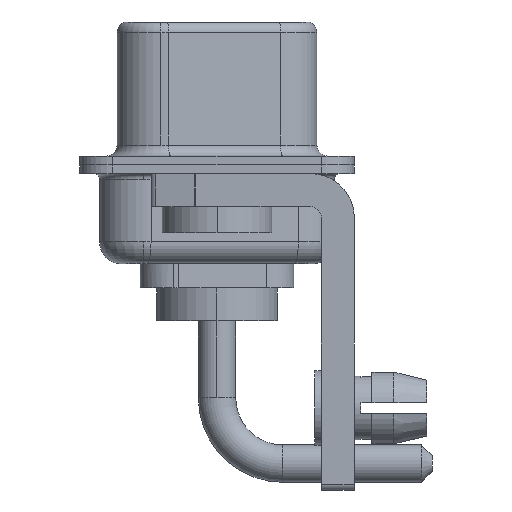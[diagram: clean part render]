
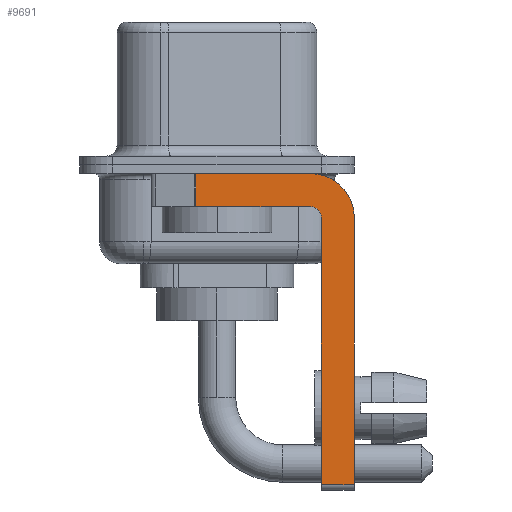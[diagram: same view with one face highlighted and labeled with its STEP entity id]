
A CAD part, left-side view. The second image highlights one B-rep face of the part: STEP entity #9691.
In plain terms, the highlighted planar face has unit normal (-1, 0, 0).
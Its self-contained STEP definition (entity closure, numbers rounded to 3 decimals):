
#87 = AXIS2_PLACEMENT_3D ( 'NONE', #12002, #17520, #7473 ) ;
#118 = AXIS2_PLACEMENT_3D ( 'NONE', #17825, #10925, #2314 ) ;
#551 = DIRECTION ( 'NONE',  ( 0., 0., 1. ) ) ;
#758 = CARTESIAN_POINT ( 'NONE',  ( -2.9, -4.25, -14.55 ) ) ;
#768 = AXIS2_PLACEMENT_3D ( 'NONE', #18091, #13930, #10912 ) ;
#1028 = CARTESIAN_POINT ( 'NONE',  ( -2.9, -6.25, -2.4 ) ) ;
#1079 = EDGE_CURVE ( 'NONE', #1593, #11810, #5171, .T. ) ;
#1318 = ORIENTED_EDGE ( 'NONE', *, *, #18041, .F. ) ;
#1593 = VERTEX_POINT ( 'NONE', #12363 ) ;
#2280 = CARTESIAN_POINT ( 'NONE',  ( -2.9, -6.25, -14.55 ) ) ;
#2314 = DIRECTION ( 'NONE',  ( 0., 0., -1. ) ) ;
#2431 = DIRECTION ( 'NONE',  ( 0., 1., 0. ) ) ;
#2499 = FACE_OUTER_BOUND ( 'NONE', #11534, .T. ) ;
#2541 = ORIENTED_EDGE ( 'NONE', *, *, #17524, .F. ) ;
#2581 = VECTOR ( 'NONE', #12455, 1000. ) ;
#2592 = VECTOR ( 'NONE', #551, 1000. ) ;
#2716 = CARTESIAN_POINT ( 'NONE',  ( -2.9, -4.25, -1.9 ) ) ;
#2843 = VERTEX_POINT ( 'NONE', #2280 ) ;
#3090 = EDGE_CURVE ( 'NONE', #16524, #1593, #5506, .T. ) ;
#3229 = EDGE_CURVE ( 'NONE', #10717, #9849, #11228, .T. ) ;
#3768 = VECTOR ( 'NONE', #11485, 1000. ) ;
#4280 = ORIENTED_EDGE ( 'NONE', *, *, #3090, .F. ) ;
#4403 = ORIENTED_EDGE ( 'NONE', *, *, #8244, .F. ) ;
#4642 = ORIENTED_EDGE ( 'NONE', *, *, #13564, .T. ) ;
#5154 = CARTESIAN_POINT ( 'NONE',  ( -2.9, 0.978, -1.9 ) ) ;
#5171 = CIRCLE ( 'NONE', #768, 2. ) ;
#5456 = VERTEX_POINT ( 'NONE', #6402 ) ;
#5506 = LINE ( 'NONE', #10982, #2581 ) ;
#5961 = CIRCLE ( 'NONE', #87, 0.5 ) ;
#6293 = PLANE ( 'NONE',  #118 ) ;
#6402 = CARTESIAN_POINT ( 'NONE',  ( -2.9, -4.75, -2.4 ) ) ;
#6850 = CARTESIAN_POINT ( 'NONE',  ( -2.9, 0.978, -1.9 ) ) ;
#7387 = CARTESIAN_POINT ( 'NONE',  ( -2.9, -4.75, -14.8 ) ) ;
#7473 = DIRECTION ( 'NONE',  ( 0., 0., 1. ) ) ;
#7584 = DIRECTION ( 'NONE',  ( 0., -1., 0. ) ) ;
#7742 = DIRECTION ( 'NONE',  ( 0., 0., -1. ) ) ;
#7865 = ORIENTED_EDGE ( 'NONE', *, *, #1079, .F. ) ;
#8244 = EDGE_CURVE ( 'NONE', #5456, #10717, #5961, .T. ) ;
#8766 = CARTESIAN_POINT ( 'NONE',  ( -2.9, -4.75, -14.55 ) ) ;
#8875 = LINE ( 'NONE', #758, #16412 ) ;
#9081 = ORIENTED_EDGE ( 'NONE', *, *, #3229, .F. ) ;
#9691 = ADVANCED_FACE ( 'NONE', ( #2499 ), #6293, .F. ) ;
#9849 = VERTEX_POINT ( 'NONE', #6850 ) ;
#10529 = LINE ( 'NONE', #7387, #2592 ) ;
#10630 = LINE ( 'NONE', #5154, #13997 ) ;
#10717 = VERTEX_POINT ( 'NONE', #16559 ) ;
#10827 = CARTESIAN_POINT ( 'NONE',  ( -2.9, 0.978, -0.4 ) ) ;
#10912 = DIRECTION ( 'NONE',  ( 0., 0., -1. ) ) ;
#10925 = DIRECTION ( 'NONE',  ( 1., 0., 0. ) ) ;
#10982 = CARTESIAN_POINT ( 'NONE',  ( -2.9, 3., -0.4 ) ) ;
#11164 = VECTOR ( 'NONE', #2431, 1000. ) ;
#11228 = LINE ( 'NONE', #2716, #11164 ) ;
#11485 = DIRECTION ( 'NONE',  ( 0., 0., -1. ) ) ;
#11534 = EDGE_LOOP ( 'NONE', ( #4280, #4642, #9081, #4403, #1318, #15178, #2541, #7865 ) ) ;
#11810 = VERTEX_POINT ( 'NONE', #1028 ) ;
#12002 = CARTESIAN_POINT ( 'NONE',  ( -2.9, -4.25, -2.4 ) ) ;
#12363 = CARTESIAN_POINT ( 'NONE',  ( -2.9, -4.25, -0.4 ) ) ;
#12455 = DIRECTION ( 'NONE',  ( 0., -1., 0. ) ) ;
#12682 = LINE ( 'NONE', #15431, #3768 ) ;
#13564 = EDGE_CURVE ( 'NONE', #16524, #9849, #10630, .T. ) ;
#13930 = DIRECTION ( 'NONE',  ( 1., 0., 0. ) ) ;
#13997 = VECTOR ( 'NONE', #7742, 1000. ) ;
#15178 = ORIENTED_EDGE ( 'NONE', *, *, #17685, .T. ) ;
#15431 = CARTESIAN_POINT ( 'NONE',  ( -2.9, -6.25, -2.4 ) ) ;
#16412 = VECTOR ( 'NONE', #7584, 1000. ) ;
#16524 = VERTEX_POINT ( 'NONE', #10827 ) ;
#16559 = CARTESIAN_POINT ( 'NONE',  ( -2.9, -4.25, -1.9 ) ) ;
#17520 = DIRECTION ( 'NONE',  ( -1., 0., 0. ) ) ;
#17524 = EDGE_CURVE ( 'NONE', #11810, #2843, #12682, .T. ) ;
#17685 = EDGE_CURVE ( 'NONE', #18042, #2843, #8875, .T. ) ;
#17825 = CARTESIAN_POINT ( 'NONE',  ( -2.9, -4.25, -2.4 ) ) ;
#18041 = EDGE_CURVE ( 'NONE', #18042, #5456, #10529, .T. ) ;
#18042 = VERTEX_POINT ( 'NONE', #8766 ) ;
#18091 = CARTESIAN_POINT ( 'NONE',  ( -2.9, -4.25, -2.4 ) ) ;
